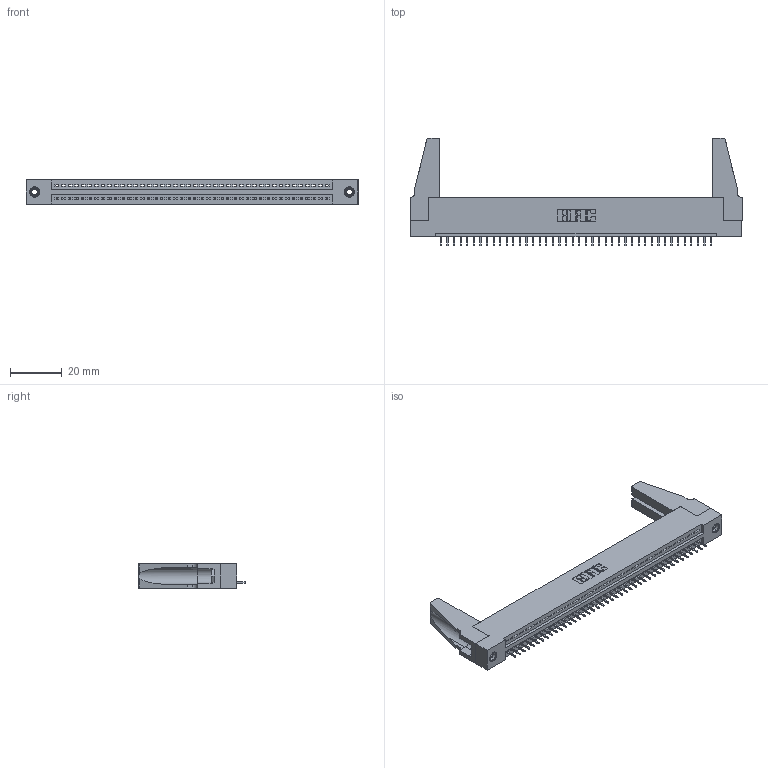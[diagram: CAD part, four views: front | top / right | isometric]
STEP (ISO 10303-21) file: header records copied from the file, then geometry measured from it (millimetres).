
FILE_DESCRIPTION (( 'STEP AP203' ), '1' );
FILE_NAME ('395-042-525-188.STEP', '2020-09-24T03:33:56', ( '' ), ( '' ), 'SwSTEP 2.0', 'SolidWorks 2020', '' );
FILE_SCHEMA (( 'CONFIG_CONTROL_DESIGN' ));
Length unit declared in the file: inch
Products named in the file (5): 395-042-525-188; 345-250-001_345-250-001-102; 345-292-001_345-293-125; 345 Part_Flush Mounting Lugs - 0.156 Dia-TH; 345-220-078_345-220-088
Assembly tree (47 placements, depth 2):
  395-042-525-188
    345 Part_Flush Mounting Lugs - 0.156 Dia-TH
    345-292-001_345-293-125  x42
    345-250-001_345-250-001-102  x2
    345-220-078_345-220-088  x2
Bounding box: 127.91 x 41.58 x 9.4 mm (x, y, z)
Volume: 15230.5 mm3; surface area: 18475 mm2
Topology: 47 solids, 47 shells, 2854 faces, 8215 edges, 5298 vertices
Faces by surface type: plane 2084, cylinder 754, cone 12, torus 4
Entity records: 33832 total; most frequent: CARTESIAN_POINT 5848, ORIENTED_EDGE 5784, DIRECTION 5116, EDGE_CURVE 2892, VECTOR 2554, LINE 2554, VERTEX_POINT 1918, AXIS2_PLACEMENT_3D 1281
